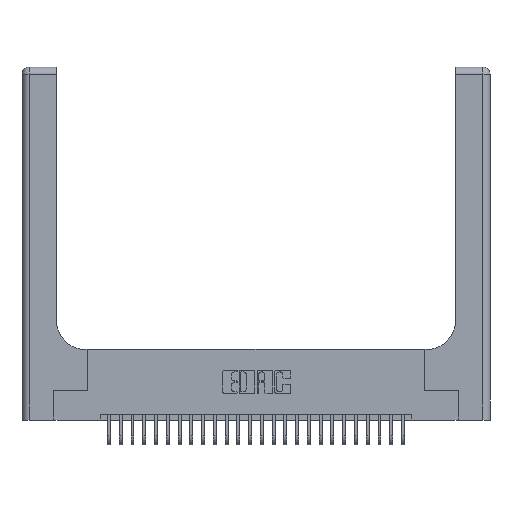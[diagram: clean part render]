
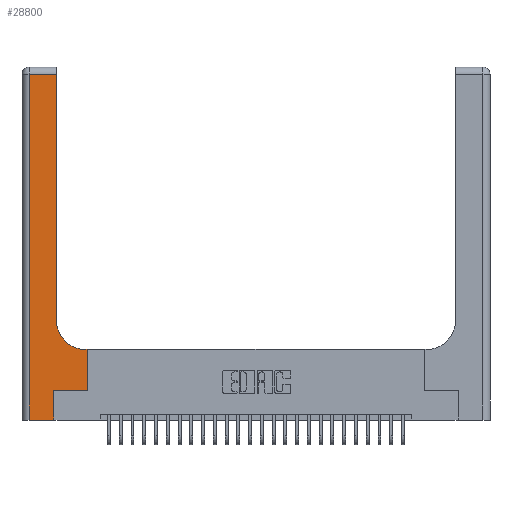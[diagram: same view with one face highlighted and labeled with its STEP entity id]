
A CAD part, top view. The second image highlights one B-rep face of the part: STEP entity #28800.
In plain terms, the highlighted planar face has unit normal (0, 0, 1).
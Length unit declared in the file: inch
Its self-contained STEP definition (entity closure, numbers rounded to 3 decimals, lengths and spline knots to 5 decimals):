
#8 = EDGE_LOOP ( 'NONE', ( #23966, #10762, #19133, #6392, #28208, #1599, #1382, #10928, #17389 ) ) ;
#974 = EDGE_CURVE ( 'NONE', #8573, #7297, #4742, .T. ) ;
#1010 = VECTOR ( 'NONE', #24226, 39.37008 ) ;
#1382 = ORIENTED_EDGE ( 'NONE', *, *, #7891, .T. ) ;
#1599 = ORIENTED_EDGE ( 'NONE', *, *, #15105, .T. ) ;
#1617 = CARTESIAN_POINT ( 'NONE',  ( 0.5415, 0.85, 0.37 ) ) ;
#1870 = VECTOR ( 'NONE', #25286, 39.37008 ) ;
#2234 = LINE ( 'NONE', #23340, #10765 ) ;
#2850 = CARTESIAN_POINT ( 'NONE',  ( 0.2915, 2.94, 0.37 ) ) ;
#3573 = VECTOR ( 'NONE', #29117, 39.37008 ) ;
#3895 = EDGE_CURVE ( 'NONE', #17417, #10016, #15362, .T. ) ;
#4742 = LINE ( 'NONE', #6678, #19950 ) ;
#4932 = DIRECTION ( 'NONE',  ( -1., 0., 0. ) ) ;
#5130 = DIRECTION ( 'NONE',  ( 0., 0., -1. ) ) ;
#5504 = EDGE_CURVE ( 'NONE', #9237, #25783, #11087, .T. ) ;
#5561 = AXIS2_PLACEMENT_3D ( 'NONE', #1617, #19775, #6221 ) ;
#6221 = DIRECTION ( 'NONE',  ( 1., 0., 0. ) ) ;
#6392 = ORIENTED_EDGE ( 'NONE', *, *, #13591, .T. ) ;
#6678 = CARTESIAN_POINT ( 'NONE',  ( 0.06, 3., 0.37 ) ) ;
#7297 = VERTEX_POINT ( 'NONE', #17068 ) ;
#7891 = EDGE_CURVE ( 'NONE', #20023, #10560, #24045, .T. ) ;
#8156 = CARTESIAN_POINT ( 'NONE',  ( 0.06, 2.94, 0.37 ) ) ;
#8292 = CARTESIAN_POINT ( 'NONE',  ( 0.2915, 3., 0.37 ) ) ;
#8573 = VERTEX_POINT ( 'NONE', #8156 ) ;
#9237 = VERTEX_POINT ( 'NONE', #29189 ) ;
#9650 = LINE ( 'NONE', #26552, #3573 ) ;
#10016 = VERTEX_POINT ( 'NONE', #16825 ) ;
#10560 = VERTEX_POINT ( 'NONE', #14029 ) ;
#10762 = ORIENTED_EDGE ( 'NONE', *, *, #21862, .T. ) ;
#10765 = VECTOR ( 'NONE', #18661, 39.37008 ) ;
#10928 = ORIENTED_EDGE ( 'NONE', *, *, #27084, .T. ) ;
#10994 = CARTESIAN_POINT ( 'NONE',  ( 0.5585, 0.25, 0.37 ) ) ;
#11087 = CIRCLE ( 'NONE', #5561, 0.25 ) ;
#11226 = DIRECTION ( 'NONE',  ( -1., 0., 0. ) ) ;
#11688 = PLANE ( 'NONE',  #28668 ) ;
#11931 = CARTESIAN_POINT ( 'NONE',  ( 0.269, 0., 0.37 ) ) ;
#13078 = CARTESIAN_POINT ( 'NONE',  ( 0., 2.94, 0.37 ) ) ;
#13591 = EDGE_CURVE ( 'NONE', #7297, #17417, #26373, .T. ) ;
#13968 = CARTESIAN_POINT ( 'NONE',  ( 0., 3., 0.37 ) ) ;
#14029 = CARTESIAN_POINT ( 'NONE',  ( 0.5585, 0.6, 0.37 ) ) ;
#14192 = LINE ( 'NONE', #8292, #1010 ) ;
#15105 = EDGE_CURVE ( 'NONE', #10016, #20023, #9650, .T. ) ;
#15362 = LINE ( 'NONE', #11931, #1870 ) ;
#15583 = VECTOR ( 'NONE', #11226, 39.37008 ) ;
#15661 = EDGE_CURVE ( 'NONE', #25783, #25270, #14192, .T. ) ;
#16461 = DIRECTION ( 'NONE',  ( 0., -1., 0. ) ) ;
#16825 = CARTESIAN_POINT ( 'NONE',  ( 0.269, 0.25, 0.37 ) ) ;
#17068 = CARTESIAN_POINT ( 'NONE',  ( 0.06, 0., 0.37 ) ) ;
#17389 = ORIENTED_EDGE ( 'NONE', *, *, #5504, .T. ) ;
#17417 = VERTEX_POINT ( 'NONE', #21867 ) ;
#18568 = CARTESIAN_POINT ( 'NONE',  ( 0.2915, 0.85, 0.37 ) ) ;
#18661 = DIRECTION ( 'NONE',  ( -1., 0., 0. ) ) ;
#19097 = DIRECTION ( 'NONE',  ( 1., 0., 0. ) ) ;
#19133 = ORIENTED_EDGE ( 'NONE', *, *, #974, .T. ) ;
#19144 = FACE_OUTER_BOUND ( 'NONE', #8, .T. ) ;
#19775 = DIRECTION ( 'NONE',  ( 0., 0., -1. ) ) ;
#19950 = VECTOR ( 'NONE', #16461, 39.37008 ) ;
#20023 = VERTEX_POINT ( 'NONE', #26060 ) ;
#21590 = LINE ( 'NONE', #13078, #15583 ) ;
#21862 = EDGE_CURVE ( 'NONE', #25270, #8573, #21590, .T. ) ;
#21867 = CARTESIAN_POINT ( 'NONE',  ( 0.269, 0., 0.37 ) ) ;
#23340 = CARTESIAN_POINT ( 'NONE',  ( 0.2915, 0.6, 0.37 ) ) ;
#23966 = ORIENTED_EDGE ( 'NONE', *, *, #15661, .T. ) ;
#24045 = LINE ( 'NONE', #10994, #25081 ) ;
#24226 = DIRECTION ( 'NONE',  ( 0., 1., 0. ) ) ;
#24938 = VECTOR ( 'NONE', #19097, 39.37008 ) ;
#25081 = VECTOR ( 'NONE', #27226, 39.37008 ) ;
#25270 = VERTEX_POINT ( 'NONE', #2850 ) ;
#25286 = DIRECTION ( 'NONE',  ( 0., 1., 0. ) ) ;
#25783 = VERTEX_POINT ( 'NONE', #18568 ) ;
#26060 = CARTESIAN_POINT ( 'NONE',  ( 0.5585, 0.25, 0.37 ) ) ;
#26373 = LINE ( 'NONE', #27868, #24938 ) ;
#26552 = CARTESIAN_POINT ( 'NONE',  ( 0.269, 0.25, 0.37 ) ) ;
#27084 = EDGE_CURVE ( 'NONE', #10560, #9237, #2234, .T. ) ;
#27226 = DIRECTION ( 'NONE',  ( 0., 1., 0. ) ) ;
#27868 = CARTESIAN_POINT ( 'NONE',  ( 0., 0., 0.37 ) ) ;
#28208 = ORIENTED_EDGE ( 'NONE', *, *, #3895, .T. ) ;
#28668 = AXIS2_PLACEMENT_3D ( 'NONE', #13968, #5130, #4932 ) ;
#28800 = ADVANCED_FACE ( 'NONE', ( #19144 ), #11688, .F. ) ;
#29117 = DIRECTION ( 'NONE',  ( 1., 0., 0. ) ) ;
#29189 = CARTESIAN_POINT ( 'NONE',  ( 0.5415, 0.6, 0.37 ) ) ;
